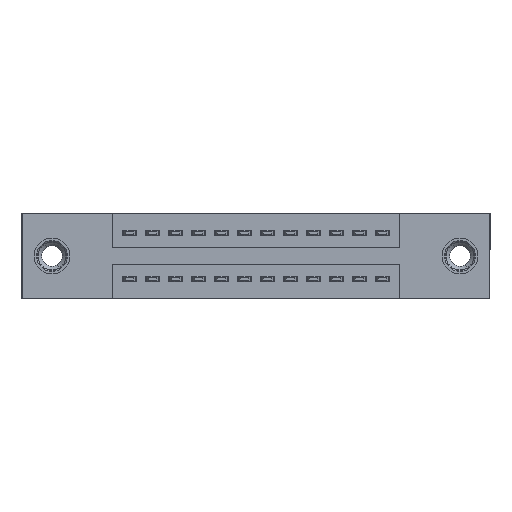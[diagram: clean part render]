
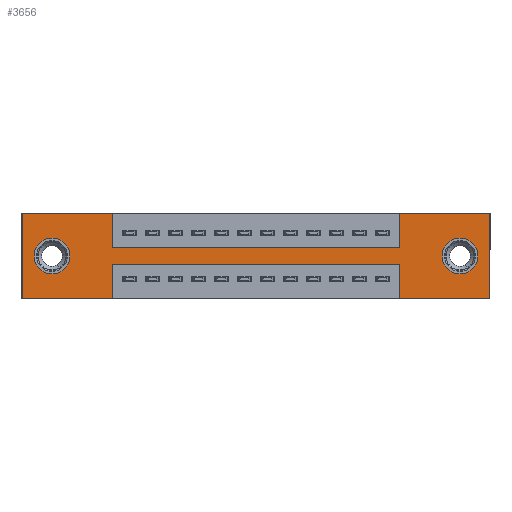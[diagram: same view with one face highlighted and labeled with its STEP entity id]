
A CAD part, front view. The second image highlights one B-rep face of the part: STEP entity #3656.
In plain terms, the highlighted planar face has unit normal (0, -1, 0).
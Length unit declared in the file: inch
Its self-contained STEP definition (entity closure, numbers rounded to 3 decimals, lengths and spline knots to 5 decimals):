
#237 = VERTEX_POINT ( 'NONE', #11044 ) ;
#290 = VECTOR ( 'NONE', #14465, 39.37008 ) ;
#377 = LINE ( 'NONE', #13430, #6166 ) ;
#436 = EDGE_CURVE ( 'NONE', #11188, #9744, #9918, .T. ) ;
#487 = CARTESIAN_POINT ( 'NONE',  ( 0., 0., 0. ) ) ;
#608 = DIRECTION ( 'NONE',  ( 0., 0., 1. ) ) ;
#640 = VECTOR ( 'NONE', #9955, 39.37008 ) ;
#745 = CARTESIAN_POINT ( 'NONE',  ( 0., 0., -0.37 ) ) ;
#812 = DIRECTION ( 'NONE',  ( 0., 0., 1. ) ) ;
#859 = CARTESIAN_POINT ( 'NONE',  ( 0., 0., 0. ) ) ;
#892 = VERTEX_POINT ( 'NONE', #2224 ) ;
#1024 = LINE ( 'NONE', #9600, #640 ) ;
#1101 = ORIENTED_EDGE ( 'NONE', *, *, #5936, .F. ) ;
#1185 = CARTESIAN_POINT ( 'NONE',  ( 2.035, 0., 0. ) ) ;
#1230 = CARTESIAN_POINT ( 'NONE',  ( 0., 0., 0. ) ) ;
#1639 = VERTEX_POINT ( 'NONE', #14764 ) ;
#1718 = CARTESIAN_POINT ( 'NONE',  ( 0.3925, 0., -0.37 ) ) ;
#1730 = DIRECTION ( 'NONE',  ( 0., 1., 0. ) ) ;
#1785 = DIRECTION ( 'NONE',  ( 1., 0., 0. ) ) ;
#1937 = DIRECTION ( 'NONE',  ( 0., 0., 1. ) ) ;
#1962 = FACE_BOUND ( 'NONE', #11953, .T. ) ;
#1991 = VECTOR ( 'NONE', #13095, 39.37008 ) ;
#2030 = CARTESIAN_POINT ( 'NONE',  ( 1.6425, 0., 0. ) ) ;
#2224 = CARTESIAN_POINT ( 'NONE',  ( 0.13, 0., -0.107 ) ) ;
#2271 = ORIENTED_EDGE ( 'NONE', *, *, #6306, .F. ) ;
#2281 = LINE ( 'NONE', #487, #14499 ) ;
#2323 = VERTEX_POINT ( 'NONE', #859 ) ;
#2361 = LINE ( 'NONE', #11346, #14937 ) ;
#2390 = CARTESIAN_POINT ( 'NONE',  ( 1.905, 0., -0.185 ) ) ;
#2464 = CARTESIAN_POINT ( 'NONE',  ( 1.6425, 0., -0.15 ) ) ;
#2597 = VERTEX_POINT ( 'NONE', #10888 ) ;
#2615 = EDGE_CURVE ( 'NONE', #14402, #2597, #1024, .T. ) ;
#2826 = VERTEX_POINT ( 'NONE', #1185 ) ;
#2864 = ORIENTED_EDGE ( 'NONE', *, *, #10691, .F. ) ;
#2963 = VECTOR ( 'NONE', #14362, 39.37008 ) ;
#3023 = VERTEX_POINT ( 'NONE', #13980 ) ;
#3139 = ORIENTED_EDGE ( 'NONE', *, *, #6834, .F. ) ;
#3411 = CARTESIAN_POINT ( 'NONE',  ( 0.3925, 0., -0.37 ) ) ;
#3433 = ORIENTED_EDGE ( 'NONE', *, *, #13986, .T. ) ;
#3648 = DIRECTION ( 'NONE',  ( 0., 0., -1. ) ) ;
#3651 = LINE ( 'NONE', #4433, #12954 ) ;
#3656 = ADVANCED_FACE ( 'NONE', ( #14207, #1962, #8388 ), #12699, .T. ) ;
#3691 = CARTESIAN_POINT ( 'NONE',  ( 0., 0., -0.37 ) ) ;
#4133 = VERTEX_POINT ( 'NONE', #1718 ) ;
#4433 = CARTESIAN_POINT ( 'NONE',  ( 0., 0., 0. ) ) ;
#4630 = DIRECTION ( 'NONE',  ( 0., 0., -1. ) ) ;
#4718 = EDGE_CURVE ( 'NONE', #1639, #11188, #377, .T. ) ;
#4948 = CARTESIAN_POINT ( 'NONE',  ( 2.035, 0., 0. ) ) ;
#4978 = EDGE_CURVE ( 'NONE', #13487, #14402, #15257, .T. ) ;
#5126 = VERTEX_POINT ( 'NONE', #7177 ) ;
#5226 = CIRCLE ( 'NONE', #14982, 0.078 ) ;
#5670 = ORIENTED_EDGE ( 'NONE', *, *, #11794, .T. ) ;
#5707 = DIRECTION ( 'NONE',  ( 0., -1., 0. ) ) ;
#5720 = CARTESIAN_POINT ( 'NONE',  ( 1.6425, 0., -0.37 ) ) ;
#5936 = EDGE_CURVE ( 'NONE', #2323, #14783, #2281, .T. ) ;
#6166 = VECTOR ( 'NONE', #6476, 39.37008 ) ;
#6306 = EDGE_CURVE ( 'NONE', #4133, #237, #10792, .T. ) ;
#6347 = EDGE_LOOP ( 'NONE', ( #3433, #5670 ) ) ;
#6476 = DIRECTION ( 'NONE',  ( 1., 0., 0. ) ) ;
#6485 = ORIENTED_EDGE ( 'NONE', *, *, #436, .F. ) ;
#6513 = VECTOR ( 'NONE', #4630, 39.37008 ) ;
#6834 = EDGE_CURVE ( 'NONE', #2826, #13856, #12390, .T. ) ;
#6855 = DIRECTION ( 'NONE',  ( 0., 1., 0. ) ) ;
#7021 = VERTEX_POINT ( 'NONE', #11167 ) ;
#7162 = EDGE_CURVE ( 'NONE', #892, #3023, #5226, .T. ) ;
#7177 = CARTESIAN_POINT ( 'NONE',  ( 1.905, 0., -0.263 ) ) ;
#7910 = DIRECTION ( 'NONE',  ( 0., 1., 0. ) ) ;
#7996 = CARTESIAN_POINT ( 'NONE',  ( 1.6425, 0., 0. ) ) ;
#8248 = EDGE_LOOP ( 'NONE', ( #11682, #9801, #10425, #8415, #3139, #2864, #6485, #13023, #10312, #1101, #11049, #2271 ) ) ;
#8388 = FACE_OUTER_BOUND ( 'NONE', #8248, .T. ) ;
#8415 = ORIENTED_EDGE ( 'NONE', *, *, #13900, .F. ) ;
#8632 = CARTESIAN_POINT ( 'NONE',  ( 0.3925, 0., 0. ) ) ;
#8636 = EDGE_CURVE ( 'NONE', #2597, #4133, #13056, .T. ) ;
#8933 = CARTESIAN_POINT ( 'NONE',  ( 0.13, 0., -0.185 ) ) ;
#9097 = LINE ( 'NONE', #8632, #13825 ) ;
#9600 = CARTESIAN_POINT ( 'NONE',  ( 0.3925, 0., -0.22 ) ) ;
#9641 = DIRECTION ( 'NONE',  ( 1., 0., 0. ) ) ;
#9661 = CIRCLE ( 'NONE', #13339, 0.078 ) ;
#9744 = VERTEX_POINT ( 'NONE', #7996 ) ;
#9801 = ORIENTED_EDGE ( 'NONE', *, *, #2615, .F. ) ;
#9805 = DIRECTION ( 'NONE',  ( 0., 0., -1. ) ) ;
#9817 = CARTESIAN_POINT ( 'NONE',  ( 0.3925, 0., 0. ) ) ;
#9918 = LINE ( 'NONE', #2030, #290 ) ;
#9955 = DIRECTION ( 'NONE',  ( -1., 0., 0. ) ) ;
#10114 = DIRECTION ( 'NONE',  ( 0., 0., 1. ) ) ;
#10215 = EDGE_CURVE ( 'NONE', #3023, #892, #12302, .T. ) ;
#10312 = ORIENTED_EDGE ( 'NONE', *, *, #14377, .F. ) ;
#10425 = ORIENTED_EDGE ( 'NONE', *, *, #4978, .F. ) ;
#10662 = ORIENTED_EDGE ( 'NONE', *, *, #7162, .T. ) ;
#10691 = EDGE_CURVE ( 'NONE', #9744, #2826, #10857, .T. ) ;
#10746 = DIRECTION ( 'NONE',  ( 0., 1., 0. ) ) ;
#10792 = LINE ( 'NONE', #3691, #1991 ) ;
#10857 = LINE ( 'NONE', #1230, #13919 ) ;
#10888 = CARTESIAN_POINT ( 'NONE',  ( 0.3925, 0., -0.22 ) ) ;
#11002 = CIRCLE ( 'NONE', #14874, 0.078 ) ;
#11044 = CARTESIAN_POINT ( 'NONE',  ( 0., 0., -0.37 ) ) ;
#11049 = ORIENTED_EDGE ( 'NONE', *, *, #12238, .F. ) ;
#11104 = ORIENTED_EDGE ( 'NONE', *, *, #10215, .T. ) ;
#11165 = AXIS2_PLACEMENT_3D ( 'NONE', #745, #5707, #13873 ) ;
#11167 = CARTESIAN_POINT ( 'NONE',  ( 1.905, 0., -0.107 ) ) ;
#11188 = VERTEX_POINT ( 'NONE', #2464 ) ;
#11311 = AXIS2_PLACEMENT_3D ( 'NONE', #8933, #1730, #10114 ) ;
#11346 = CARTESIAN_POINT ( 'NONE',  ( 0., 0., -0.37 ) ) ;
#11682 = ORIENTED_EDGE ( 'NONE', *, *, #8636, .F. ) ;
#11695 = CARTESIAN_POINT ( 'NONE',  ( 1.6425, 0., -0.37 ) ) ;
#11794 = EDGE_CURVE ( 'NONE', #5126, #7021, #11002, .T. ) ;
#11803 = VECTOR ( 'NONE', #812, 39.37008 ) ;
#11953 = EDGE_LOOP ( 'NONE', ( #10662, #11104 ) ) ;
#12135 = CARTESIAN_POINT ( 'NONE',  ( 1.6425, 0., -0.22 ) ) ;
#12238 = EDGE_CURVE ( 'NONE', #237, #2323, #3651, .T. ) ;
#12302 = CIRCLE ( 'NONE', #11311, 0.078 ) ;
#12390 = LINE ( 'NONE', #4948, #2963 ) ;
#12494 = DIRECTION ( 'NONE',  ( -1., 0., 0. ) ) ;
#12699 = PLANE ( 'NONE',  #11165 ) ;
#12954 = VECTOR ( 'NONE', #1937, 39.37008 ) ;
#13023 = ORIENTED_EDGE ( 'NONE', *, *, #4718, .F. ) ;
#13056 = LINE ( 'NONE', #3411, #6513 ) ;
#13095 = DIRECTION ( 'NONE',  ( -1., 0., 0. ) ) ;
#13339 = AXIS2_PLACEMENT_3D ( 'NONE', #13816, #6855, #14991 ) ;
#13430 = CARTESIAN_POINT ( 'NONE',  ( 0.3925, 0., -0.15 ) ) ;
#13487 = VERTEX_POINT ( 'NONE', #11695 ) ;
#13816 = CARTESIAN_POINT ( 'NONE',  ( 1.905, 0., -0.185 ) ) ;
#13825 = VECTOR ( 'NONE', #9805, 39.37008 ) ;
#13856 = VERTEX_POINT ( 'NONE', #14734 ) ;
#13873 = DIRECTION ( 'NONE',  ( 0., 0., -1. ) ) ;
#13900 = EDGE_CURVE ( 'NONE', #13856, #13487, #2361, .T. ) ;
#13919 = VECTOR ( 'NONE', #9641, 39.37008 ) ;
#13980 = CARTESIAN_POINT ( 'NONE',  ( 0.13, 0., -0.263 ) ) ;
#13986 = EDGE_CURVE ( 'NONE', #7021, #5126, #9661, .T. ) ;
#14207 = FACE_BOUND ( 'NONE', #6347, .T. ) ;
#14362 = DIRECTION ( 'NONE',  ( 0., 0., -1. ) ) ;
#14377 = EDGE_CURVE ( 'NONE', #14783, #1639, #9097, .T. ) ;
#14402 = VERTEX_POINT ( 'NONE', #12135 ) ;
#14465 = DIRECTION ( 'NONE',  ( 0., 0., 1. ) ) ;
#14499 = VECTOR ( 'NONE', #1785, 39.37008 ) ;
#14734 = CARTESIAN_POINT ( 'NONE',  ( 2.035, 0., -0.37 ) ) ;
#14764 = CARTESIAN_POINT ( 'NONE',  ( 0.3925, 0., -0.15 ) ) ;
#14783 = VERTEX_POINT ( 'NONE', #9817 ) ;
#14856 = CARTESIAN_POINT ( 'NONE',  ( 0.13, 0., -0.185 ) ) ;
#14874 = AXIS2_PLACEMENT_3D ( 'NONE', #2390, #10746, #3648 ) ;
#14937 = VECTOR ( 'NONE', #12494, 39.37008 ) ;
#14982 = AXIS2_PLACEMENT_3D ( 'NONE', #14856, #7910, #608 ) ;
#14991 = DIRECTION ( 'NONE',  ( 0., 0., -1. ) ) ;
#15257 = LINE ( 'NONE', #5720, #11803 ) ;
